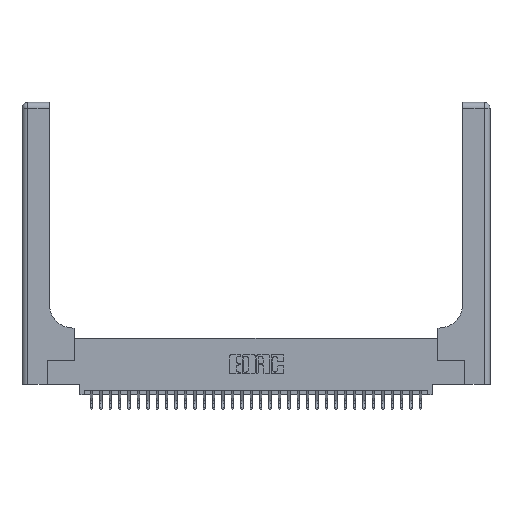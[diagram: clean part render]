
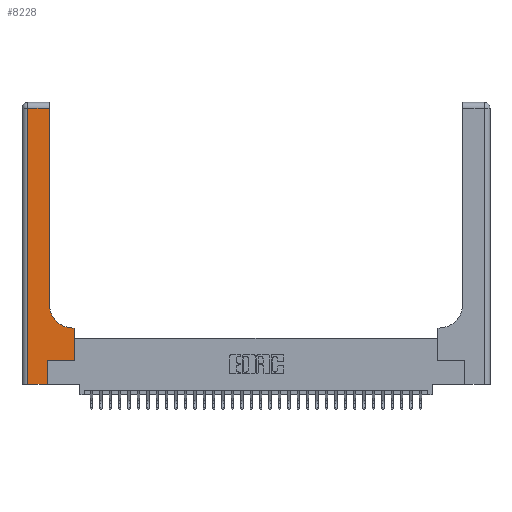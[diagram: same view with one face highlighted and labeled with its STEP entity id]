
A CAD part, top view. The second image highlights one B-rep face of the part: STEP entity #8228.
In plain terms, the highlighted planar face has unit normal (0, 0, 1).
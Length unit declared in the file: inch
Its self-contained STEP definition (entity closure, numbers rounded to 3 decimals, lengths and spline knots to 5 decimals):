
#481 = VERTEX_POINT ( 'NONE', #5076 ) ;
#880 = EDGE_CURVE ( 'NONE', #1199, #23029, #22798, .T. ) ;
#1199 = VERTEX_POINT ( 'NONE', #22045 ) ;
#1751 = DIRECTION ( 'NONE',  ( 0., 0., -1. ) ) ;
#1846 = FACE_OUTER_BOUND ( 'NONE', #4188, .T. ) ;
#2947 = DIRECTION ( 'NONE',  ( 0., 0., -1. ) ) ;
#3028 = VECTOR ( 'NONE', #22730, 39.37008 ) ;
#3647 = CARTESIAN_POINT ( 'NONE',  ( 0., 0., 0.37 ) ) ;
#3699 = ORIENTED_EDGE ( 'NONE', *, *, #8715, .T. ) ;
#3763 = CARTESIAN_POINT ( 'NONE',  ( 0.5415, 0.6, 0.37 ) ) ;
#4188 = EDGE_LOOP ( 'NONE', ( #3699, #14310, #24683, #33344, #10090, #32966, #7141, #31361, #11828 ) ) ;
#4956 = LINE ( 'NONE', #3647, #33300 ) ;
#5063 = LINE ( 'NONE', #19539, #33384 ) ;
#5076 = CARTESIAN_POINT ( 'NONE',  ( 0.2915, 2.94, 0.37 ) ) ;
#5992 = EDGE_CURVE ( 'NONE', #11129, #14074, #5063, .T. ) ;
#7141 = ORIENTED_EDGE ( 'NONE', *, *, #880, .T. ) ;
#7371 = EDGE_CURVE ( 'NONE', #10418, #11129, #4956, .T. ) ;
#8228 = ADVANCED_FACE ( 'NONE', ( #1846 ), #28510, .F. ) ;
#8305 = CARTESIAN_POINT ( 'NONE',  ( 0., 2.94, 0.37 ) ) ;
#8544 = CARTESIAN_POINT ( 'NONE',  ( 0.06, 2.94, 0.37 ) ) ;
#8715 = EDGE_CURVE ( 'NONE', #9928, #481, #22498, .T. ) ;
#9928 = VERTEX_POINT ( 'NONE', #27845 ) ;
#10090 = ORIENTED_EDGE ( 'NONE', *, *, #5992, .T. ) ;
#10418 = VERTEX_POINT ( 'NONE', #32376 ) ;
#10592 = VERTEX_POINT ( 'NONE', #3763 ) ;
#11129 = VERTEX_POINT ( 'NONE', #14034 ) ;
#11592 = VECTOR ( 'NONE', #17402, 39.37008 ) ;
#11828 = ORIENTED_EDGE ( 'NONE', *, *, #32246, .T. ) ;
#13057 = AXIS2_PLACEMENT_3D ( 'NONE', #19132, #2947, #21804 ) ;
#13796 = EDGE_CURVE ( 'NONE', #23029, #10592, #29343, .T. ) ;
#13886 = CARTESIAN_POINT ( 'NONE',  ( 0.269, 0.25, 0.37 ) ) ;
#14034 = CARTESIAN_POINT ( 'NONE',  ( 0.269, 0., 0.37 ) ) ;
#14074 = VERTEX_POINT ( 'NONE', #27501 ) ;
#14310 = ORIENTED_EDGE ( 'NONE', *, *, #22099, .T. ) ;
#14965 = LINE ( 'NONE', #13886, #28241 ) ;
#17200 = EDGE_CURVE ( 'NONE', #14074, #1199, #14965, .T. ) ;
#17402 = DIRECTION ( 'NONE',  ( 0., -1., 0. ) ) ;
#18861 = VECTOR ( 'NONE', #21652, 39.37008 ) ;
#19132 = CARTESIAN_POINT ( 'NONE',  ( 0.5415, 0.85, 0.37 ) ) ;
#19539 = CARTESIAN_POINT ( 'NONE',  ( 0.269, 0., 0.37 ) ) ;
#19719 = LINE ( 'NONE', #8305, #18861 ) ;
#19748 = AXIS2_PLACEMENT_3D ( 'NONE', #33773, #1751, #20632 ) ;
#19791 = DIRECTION ( 'NONE',  ( 1., 0., 0. ) ) ;
#20632 = DIRECTION ( 'NONE',  ( -1., 0., 0. ) ) ;
#21467 = VECTOR ( 'NONE', #31903, 39.37008 ) ;
#21652 = DIRECTION ( 'NONE',  ( -1., 0., 0. ) ) ;
#21665 = VECTOR ( 'NONE', #25130, 39.37008 ) ;
#21804 = DIRECTION ( 'NONE',  ( 1., 0., 0. ) ) ;
#21852 = CIRCLE ( 'NONE', #13057, 0.25 ) ;
#22045 = CARTESIAN_POINT ( 'NONE',  ( 0.5585, 0.25, 0.37 ) ) ;
#22099 = EDGE_CURVE ( 'NONE', #481, #28859, #19719, .T. ) ;
#22489 = CARTESIAN_POINT ( 'NONE',  ( 0.2915, 3., 0.37 ) ) ;
#22498 = LINE ( 'NONE', #22489, #21665 ) ;
#22730 = DIRECTION ( 'NONE',  ( 0., 1., 0. ) ) ;
#22798 = LINE ( 'NONE', #27945, #3028 ) ;
#23029 = VERTEX_POINT ( 'NONE', #23186 ) ;
#23186 = CARTESIAN_POINT ( 'NONE',  ( 0.5585, 0.6, 0.37 ) ) ;
#23898 = CARTESIAN_POINT ( 'NONE',  ( 0.2915, 0.6, 0.37 ) ) ;
#24683 = ORIENTED_EDGE ( 'NONE', *, *, #26266, .T. ) ;
#24729 = DIRECTION ( 'NONE',  ( 0., 1., 0. ) ) ;
#25130 = DIRECTION ( 'NONE',  ( 0., 1., 0. ) ) ;
#26266 = EDGE_CURVE ( 'NONE', #28859, #10418, #30327, .T. ) ;
#27114 = DIRECTION ( 'NONE',  ( 1., 0., 0. ) ) ;
#27501 = CARTESIAN_POINT ( 'NONE',  ( 0.269, 0.25, 0.37 ) ) ;
#27845 = CARTESIAN_POINT ( 'NONE',  ( 0.2915, 0.85, 0.37 ) ) ;
#27945 = CARTESIAN_POINT ( 'NONE',  ( 0.5585, 0.25, 0.37 ) ) ;
#28241 = VECTOR ( 'NONE', #27114, 39.37008 ) ;
#28510 = PLANE ( 'NONE',  #19748 ) ;
#28859 = VERTEX_POINT ( 'NONE', #8544 ) ;
#29343 = LINE ( 'NONE', #23898, #21467 ) ;
#30327 = LINE ( 'NONE', #33252, #11592 ) ;
#31361 = ORIENTED_EDGE ( 'NONE', *, *, #13796, .T. ) ;
#31903 = DIRECTION ( 'NONE',  ( -1., 0., 0. ) ) ;
#32246 = EDGE_CURVE ( 'NONE', #10592, #9928, #21852, .T. ) ;
#32376 = CARTESIAN_POINT ( 'NONE',  ( 0.06, 0., 0.37 ) ) ;
#32966 = ORIENTED_EDGE ( 'NONE', *, *, #17200, .T. ) ;
#33252 = CARTESIAN_POINT ( 'NONE',  ( 0.06, 3., 0.37 ) ) ;
#33300 = VECTOR ( 'NONE', #19791, 39.37008 ) ;
#33344 = ORIENTED_EDGE ( 'NONE', *, *, #7371, .T. ) ;
#33384 = VECTOR ( 'NONE', #24729, 39.37008 ) ;
#33773 = CARTESIAN_POINT ( 'NONE',  ( 0., 3., 0.37 ) ) ;
